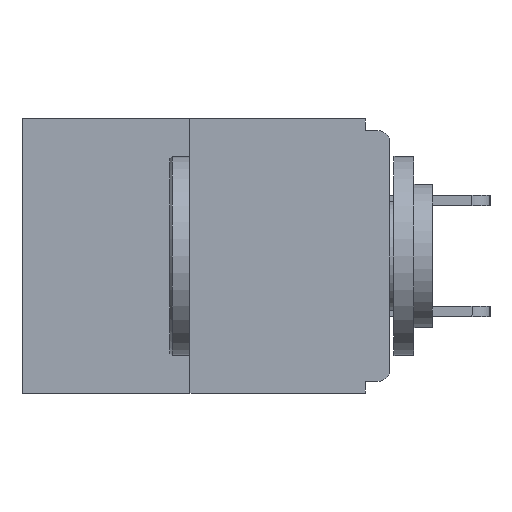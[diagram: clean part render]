
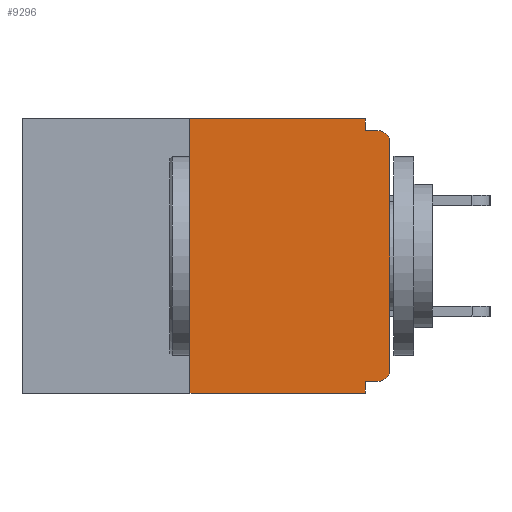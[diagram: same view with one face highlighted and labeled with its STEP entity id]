
A CAD part, left-side view. The second image highlights one B-rep face of the part: STEP entity #9296.
In plain terms, the highlighted planar face has unit normal (-1, 0, 0).
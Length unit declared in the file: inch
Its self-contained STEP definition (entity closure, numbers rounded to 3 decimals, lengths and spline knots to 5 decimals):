
#10 = CARTESIAN_POINT ( 'NONE',  ( 0., 0.46, 0. ) ) ;
#147 = CARTESIAN_POINT ( 'NONE',  ( 0., 0.031, -0.343 ) ) ;
#650 = EDGE_CURVE ( 'NONE', #8864, #12191, #3635, .T. ) ;
#786 = CARTESIAN_POINT ( 'NONE',  ( 0., 0., -0.328 ) ) ;
#876 = CARTESIAN_POINT ( 'NONE',  ( 0., 0.031, -0.328 ) ) ;
#893 = CARTESIAN_POINT ( 'NONE',  ( 0., 0., 0. ) ) ;
#954 = VERTEX_POINT ( 'NONE', #6177 ) ;
#963 = AXIS2_PLACEMENT_3D ( 'NONE', #3555, #12606, #9475 ) ;
#1035 = EDGE_CURVE ( 'NONE', #11501, #12158, #7662, .T. ) ;
#1046 = DIRECTION ( 'NONE',  ( 0., 1., 0. ) ) ;
#1067 = DIRECTION ( 'NONE',  ( 0., 0., -1. ) ) ;
#1070 = DIRECTION ( 'NONE',  ( 0., 0., -1. ) ) ;
#1345 = CARTESIAN_POINT ( 'NONE',  ( 0., 0.031, -0.343 ) ) ;
#1389 = LINE ( 'NONE', #893, #5856 ) ;
#1407 = DIRECTION ( 'NONE',  ( 0., -1., 0. ) ) ;
#1487 = CARTESIAN_POINT ( 'NONE',  ( 0., 0.25, -0.343 ) ) ;
#2159 = VECTOR ( 'NONE', #1046, 39.37008 ) ;
#2209 = VERTEX_POINT ( 'NONE', #11803 ) ;
#2506 = ORIENTED_EDGE ( 'NONE', *, *, #4347, .T. ) ;
#2624 = VECTOR ( 'NONE', #4719, 39.37008 ) ;
#2829 = DIRECTION ( 'NONE',  ( 0., 0., 1. ) ) ;
#3025 = ORIENTED_EDGE ( 'NONE', *, *, #12549, .T. ) ;
#3555 = CARTESIAN_POINT ( 'NONE',  ( 0., 0.015, -0.03 ) ) ;
#3603 = CARTESIAN_POINT ( 'NONE',  ( 0., 0.25, 0. ) ) ;
#3635 = LINE ( 'NONE', #12725, #5504 ) ;
#3889 = DIRECTION ( 'NONE',  ( 1., 0., 0. ) ) ;
#3944 = ORIENTED_EDGE ( 'NONE', *, *, #12537, .F. ) ;
#3985 = EDGE_CURVE ( 'NONE', #954, #2209, #4994, .T. ) ;
#4161 = CARTESIAN_POINT ( 'NONE',  ( 0., 0.015, -0.328 ) ) ;
#4238 = ORIENTED_EDGE ( 'NONE', *, *, #650, .T. ) ;
#4347 = EDGE_CURVE ( 'NONE', #11992, #2209, #4685, .T. ) ;
#4451 = ORIENTED_EDGE ( 'NONE', *, *, #1035, .F. ) ;
#4505 = DIRECTION ( 'NONE',  ( 0., 0., -1. ) ) ;
#4640 = ORIENTED_EDGE ( 'NONE', *, *, #3985, .F. ) ;
#4685 = CIRCLE ( 'NONE', #963, 0.015 ) ;
#4719 = DIRECTION ( 'NONE',  ( 0., 0., -1. ) ) ;
#4888 = CARTESIAN_POINT ( 'NONE',  ( 0., 0.25, 0. ) ) ;
#4908 = DIRECTION ( 'NONE',  ( 0., 0., 1. ) ) ;
#4921 = LINE ( 'NONE', #147, #9279 ) ;
#4994 = LINE ( 'NONE', #6199, #7041 ) ;
#5504 = VECTOR ( 'NONE', #7852, 39.37008 ) ;
#5606 = CARTESIAN_POINT ( 'NONE',  ( 0., 0.031, 0. ) ) ;
#5856 = VECTOR ( 'NONE', #4908, 39.37008 ) ;
#5979 = PLANE ( 'NONE',  #11308 ) ;
#6177 = CARTESIAN_POINT ( 'NONE',  ( 0., 0.031, -0.015 ) ) ;
#6199 = CARTESIAN_POINT ( 'NONE',  ( 0., 0., -0.015 ) ) ;
#6392 = EDGE_CURVE ( 'NONE', #8864, #11501, #10215, .T. ) ;
#6748 = VECTOR ( 'NONE', #12246, 39.37008 ) ;
#6755 = ORIENTED_EDGE ( 'NONE', *, *, #12312, .F. ) ;
#6828 = LINE ( 'NONE', #786, #2159 ) ;
#7041 = VECTOR ( 'NONE', #1407, 39.37008 ) ;
#7066 = ORIENTED_EDGE ( 'NONE', *, *, #6392, .F. ) ;
#7254 = EDGE_CURVE ( 'NONE', #11207, #8966, #6828, .T. ) ;
#7662 = LINE ( 'NONE', #12287, #6748 ) ;
#7852 = DIRECTION ( 'NONE',  ( 0., -1., 0. ) ) ;
#8060 = DIRECTION ( 'NONE',  ( -1., 0., 0. ) ) ;
#8387 = CARTESIAN_POINT ( 'NONE',  ( 0., 0., -0.03 ) ) ;
#8463 = AXIS2_PLACEMENT_3D ( 'NONE', #9996, #8060, #1070 ) ;
#8864 = VERTEX_POINT ( 'NONE', #1487 ) ;
#8966 = VERTEX_POINT ( 'NONE', #876 ) ;
#9065 = CARTESIAN_POINT ( 'NONE',  ( 0., 0.031, 0. ) ) ;
#9279 = VECTOR ( 'NONE', #4505, 39.37008 ) ;
#9296 = ADVANCED_FACE ( 'NONE', ( #9513 ), #5979, .F. ) ;
#9426 = ORIENTED_EDGE ( 'NONE', *, *, #7254, .F. ) ;
#9475 = DIRECTION ( 'NONE',  ( 0., 0., -1. ) ) ;
#9513 = FACE_OUTER_BOUND ( 'NONE', #9783, .T. ) ;
#9783 = EDGE_LOOP ( 'NONE', ( #4451, #7066, #4238, #3944, #9426, #11053, #3025, #2506, #4640, #6755 ) ) ;
#9996 = CARTESIAN_POINT ( 'NONE',  ( 0., 0.015, -0.313 ) ) ;
#10215 = LINE ( 'NONE', #4888, #11292 ) ;
#10409 = EDGE_CURVE ( 'NONE', #11207, #12705, #10846, .T. ) ;
#10846 = CIRCLE ( 'NONE', #8463, 0.015 ) ;
#11053 = ORIENTED_EDGE ( 'NONE', *, *, #10409, .T. ) ;
#11207 = VERTEX_POINT ( 'NONE', #4161 ) ;
#11292 = VECTOR ( 'NONE', #2829, 39.37008 ) ;
#11308 = AXIS2_PLACEMENT_3D ( 'NONE', #10, #3889, #1067 ) ;
#11501 = VERTEX_POINT ( 'NONE', #3603 ) ;
#11803 = CARTESIAN_POINT ( 'NONE',  ( 0., 0.015, -0.015 ) ) ;
#11992 = VERTEX_POINT ( 'NONE', #8387 ) ;
#12030 = LINE ( 'NONE', #5606, #2624 ) ;
#12158 = VERTEX_POINT ( 'NONE', #9065 ) ;
#12191 = VERTEX_POINT ( 'NONE', #1345 ) ;
#12246 = DIRECTION ( 'NONE',  ( 0., -1., 0. ) ) ;
#12287 = CARTESIAN_POINT ( 'NONE',  ( 0., 0.46, 0. ) ) ;
#12306 = CARTESIAN_POINT ( 'NONE',  ( 0., 0., -0.313 ) ) ;
#12312 = EDGE_CURVE ( 'NONE', #12158, #954, #12030, .T. ) ;
#12537 = EDGE_CURVE ( 'NONE', #8966, #12191, #4921, .T. ) ;
#12549 = EDGE_CURVE ( 'NONE', #12705, #11992, #1389, .T. ) ;
#12606 = DIRECTION ( 'NONE',  ( -1., 0., 0. ) ) ;
#12705 = VERTEX_POINT ( 'NONE', #12306 ) ;
#12725 = CARTESIAN_POINT ( 'NONE',  ( 0., 0.46, -0.343 ) ) ;
